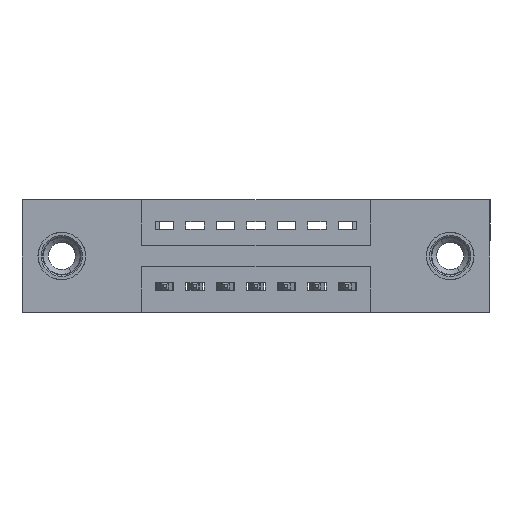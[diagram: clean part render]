
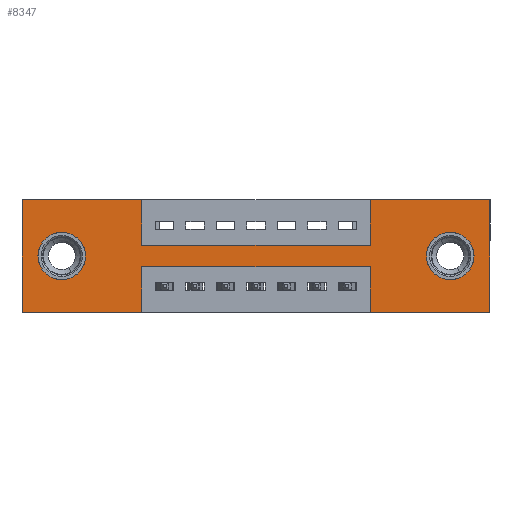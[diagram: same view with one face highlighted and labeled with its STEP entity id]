
A CAD part, front view. The second image highlights one B-rep face of the part: STEP entity #8347.
In plain terms, the highlighted planar face has unit normal (0, -1, 0).
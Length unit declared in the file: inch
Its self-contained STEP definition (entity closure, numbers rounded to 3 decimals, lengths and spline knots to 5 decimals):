
#15 = CARTESIAN_POINT ( 'NONE',  ( 1.405, 0., -0.263 ) ) ;
#103 = CARTESIAN_POINT ( 'NONE',  ( 1.1425, 0., -0.37 ) ) ;
#186 = DIRECTION ( 'NONE',  ( 0., 0., 1. ) ) ;
#274 = CARTESIAN_POINT ( 'NONE',  ( 1.1425, 0., -0.22 ) ) ;
#334 = DIRECTION ( 'NONE',  ( 0., 1., 0. ) ) ;
#341 = DIRECTION ( 'NONE',  ( 0., 1., 0. ) ) ;
#422 = CARTESIAN_POINT ( 'NONE',  ( 1.405, 0., -0.185 ) ) ;
#465 = DIRECTION ( 'NONE',  ( 0., 1., 0. ) ) ;
#527 = ORIENTED_EDGE ( 'NONE', *, *, #3583, .F. ) ;
#692 = VERTEX_POINT ( 'NONE', #10592 ) ;
#693 = ORIENTED_EDGE ( 'NONE', *, *, #2341, .F. ) ;
#712 = ORIENTED_EDGE ( 'NONE', *, *, #7673, .F. ) ;
#758 = DIRECTION ( 'NONE',  ( -1., 0., 0. ) ) ;
#780 = ORIENTED_EDGE ( 'NONE', *, *, #11427, .F. ) ;
#804 = ORIENTED_EDGE ( 'NONE', *, *, #12140, .F. ) ;
#953 = VECTOR ( 'NONE', #7619, 39.37008 ) ;
#972 = CARTESIAN_POINT ( 'NONE',  ( 0., 0., 0. ) ) ;
#1027 = DIRECTION ( 'NONE',  ( 0., 0., -1. ) ) ;
#1092 = ORIENTED_EDGE ( 'NONE', *, *, #7418, .T. ) ;
#1147 = VERTEX_POINT ( 'NONE', #6184 ) ;
#1318 = VERTEX_POINT ( 'NONE', #2509 ) ;
#1420 = ORIENTED_EDGE ( 'NONE', *, *, #5112, .F. ) ;
#1443 = CARTESIAN_POINT ( 'NONE',  ( 0.13, 0., -0.185 ) ) ;
#1456 = AXIS2_PLACEMENT_3D ( 'NONE', #2795, #9388, #11253 ) ;
#1524 = LINE ( 'NONE', #972, #10943 ) ;
#1564 = DIRECTION ( 'NONE',  ( -1., 0., 0. ) ) ;
#1749 = EDGE_CURVE ( 'NONE', #9390, #4293, #10101, .T. ) ;
#1927 = DIRECTION ( 'NONE',  ( 1., 0., 0. ) ) ;
#1957 = CARTESIAN_POINT ( 'NONE',  ( 0., 0., 0. ) ) ;
#1993 = LINE ( 'NONE', #1957, #953 ) ;
#2012 = LINE ( 'NONE', #10141, #4493 ) ;
#2042 = CARTESIAN_POINT ( 'NONE',  ( 0.3925, 0., -0.37 ) ) ;
#2138 = CARTESIAN_POINT ( 'NONE',  ( 1.1425, 0., -0.37 ) ) ;
#2214 = LINE ( 'NONE', #8931, #7953 ) ;
#2218 = ORIENTED_EDGE ( 'NONE', *, *, #7814, .T. ) ;
#2341 = EDGE_CURVE ( 'NONE', #6186, #4731, #8759, .T. ) ;
#2509 = CARTESIAN_POINT ( 'NONE',  ( 0.3925, 0., -0.15 ) ) ;
#2535 = CARTESIAN_POINT ( 'NONE',  ( 0., 0., -0.37 ) ) ;
#2539 = CARTESIAN_POINT ( 'NONE',  ( 1.1425, 0., 0. ) ) ;
#2795 = CARTESIAN_POINT ( 'NONE',  ( 0., 0., -0.37 ) ) ;
#2875 = VECTOR ( 'NONE', #8533, 39.37008 ) ;
#2930 = EDGE_LOOP ( 'NONE', ( #6854, #8489, #693, #527, #804, #712, #3038, #780, #1420, #8647, #11917, #7515 ) ) ;
#3038 = ORIENTED_EDGE ( 'NONE', *, *, #9083, .F. ) ;
#3223 = CARTESIAN_POINT ( 'NONE',  ( 0.13, 0., -0.185 ) ) ;
#3583 = EDGE_CURVE ( 'NONE', #1147, #6186, #9122, .T. ) ;
#3720 = CARTESIAN_POINT ( 'NONE',  ( 0., 0., -0.37 ) ) ;
#3762 = CARTESIAN_POINT ( 'NONE',  ( 1.535, 0., 0. ) ) ;
#4062 = LINE ( 'NONE', #7671, #9357 ) ;
#4078 = DIRECTION ( 'NONE',  ( 0., 0., 1. ) ) ;
#4095 = EDGE_CURVE ( 'NONE', #9606, #11121, #4566, .T. ) ;
#4162 = CIRCLE ( 'NONE', #8846, 0.078 ) ;
#4177 = CIRCLE ( 'NONE', #8293, 0.078 ) ;
#4293 = VERTEX_POINT ( 'NONE', #7997 ) ;
#4306 = DIRECTION ( 'NONE',  ( 0., 0., -1. ) ) ;
#4493 = VECTOR ( 'NONE', #758, 39.37008 ) ;
#4566 = CIRCLE ( 'NONE', #11667, 0.078 ) ;
#4603 = LINE ( 'NONE', #12172, #8989 ) ;
#4631 = DIRECTION ( 'NONE',  ( 0., 0., 1. ) ) ;
#4708 = VERTEX_POINT ( 'NONE', #15 ) ;
#4731 = VERTEX_POINT ( 'NONE', #274 ) ;
#4895 = CARTESIAN_POINT ( 'NONE',  ( 0.3925, 0., -0.22 ) ) ;
#5112 = EDGE_CURVE ( 'NONE', #5914, #1318, #6029, .T. ) ;
#5321 = CARTESIAN_POINT ( 'NONE',  ( 0., 0., 0. ) ) ;
#5438 = CARTESIAN_POINT ( 'NONE',  ( 0., 0., 0. ) ) ;
#5441 = VECTOR ( 'NONE', #1564, 39.37008 ) ;
#5484 = CARTESIAN_POINT ( 'NONE',  ( 1.1425, 0., -0.15 ) ) ;
#5727 = VECTOR ( 'NONE', #1027, 39.37008 ) ;
#5738 = LINE ( 'NONE', #3762, #8076 ) ;
#5914 = VERTEX_POINT ( 'NONE', #10557 ) ;
#5963 = VECTOR ( 'NONE', #186, 39.37008 ) ;
#5968 = CARTESIAN_POINT ( 'NONE',  ( 1.405, 0., -0.185 ) ) ;
#6029 = LINE ( 'NONE', #8507, #5727 ) ;
#6184 = CARTESIAN_POINT ( 'NONE',  ( 1.535, 0., -0.37 ) ) ;
#6186 = VERTEX_POINT ( 'NONE', #2138 ) ;
#6219 = CARTESIAN_POINT ( 'NONE',  ( 0.13, 0., -0.107 ) ) ;
#6510 = EDGE_CURVE ( 'NONE', #4731, #9714, #2012, .T. ) ;
#6512 = FACE_OUTER_BOUND ( 'NONE', #2930, .T. ) ;
#6676 = EDGE_CURVE ( 'NONE', #9714, #9390, #4062, .T. ) ;
#6747 = EDGE_LOOP ( 'NONE', ( #1092, #8422 ) ) ;
#6854 = ORIENTED_EDGE ( 'NONE', *, *, #6676, .F. ) ;
#7052 = VERTEX_POINT ( 'NONE', #5321 ) ;
#7059 = EDGE_CURVE ( 'NONE', #4293, #7052, #7744, .T. ) ;
#7104 = FACE_BOUND ( 'NONE', #11002, .T. ) ;
#7418 = EDGE_CURVE ( 'NONE', #11121, #9606, #4177, .T. ) ;
#7469 = PLANE ( 'NONE',  #1456 ) ;
#7515 = ORIENTED_EDGE ( 'NONE', *, *, #1749, .F. ) ;
#7619 = DIRECTION ( 'NONE',  ( 1., 0., 0. ) ) ;
#7671 = CARTESIAN_POINT ( 'NONE',  ( 0.3925, 0., -0.37 ) ) ;
#7673 = EDGE_CURVE ( 'NONE', #11431, #11813, #1993, .T. ) ;
#7744 = LINE ( 'NONE', #5438, #9032 ) ;
#7814 = EDGE_CURVE ( 'NONE', #692, #4708, #4162, .T. ) ;
#7857 = DIRECTION ( 'NONE',  ( 0., 0., -1. ) ) ;
#7920 = EDGE_CURVE ( 'NONE', #7052, #5914, #1524, .T. ) ;
#7953 = VECTOR ( 'NONE', #10803, 39.37008 ) ;
#7983 = CARTESIAN_POINT ( 'NONE',  ( 0.13, 0., -0.263 ) ) ;
#7997 = CARTESIAN_POINT ( 'NONE',  ( 0., 0., -0.37 ) ) ;
#8076 = VECTOR ( 'NONE', #9401, 39.37008 ) ;
#8293 = AXIS2_PLACEMENT_3D ( 'NONE', #1443, #341, #4078 ) ;
#8347 = ADVANCED_FACE ( 'NONE', ( #7104, #10488, #6512 ), #7469, .T. ) ;
#8422 = ORIENTED_EDGE ( 'NONE', *, *, #4095, .T. ) ;
#8489 = ORIENTED_EDGE ( 'NONE', *, *, #6510, .F. ) ;
#8507 = CARTESIAN_POINT ( 'NONE',  ( 0.3925, 0., 0. ) ) ;
#8533 = DIRECTION ( 'NONE',  ( -1., 0., 0. ) ) ;
#8647 = ORIENTED_EDGE ( 'NONE', *, *, #7920, .F. ) ;
#8759 = LINE ( 'NONE', #103, #5963 ) ;
#8846 = AXIS2_PLACEMENT_3D ( 'NONE', #422, #465, #4306 ) ;
#8931 = CARTESIAN_POINT ( 'NONE',  ( 0.3925, 0., -0.15 ) ) ;
#8989 = VECTOR ( 'NONE', #4631, 39.37008 ) ;
#9032 = VECTOR ( 'NONE', #12021, 39.37008 ) ;
#9083 = EDGE_CURVE ( 'NONE', #12078, #11431, #4603, .T. ) ;
#9122 = LINE ( 'NONE', #2535, #5441 ) ;
#9310 = CIRCLE ( 'NONE', #11406, 0.078 ) ;
#9357 = VECTOR ( 'NONE', #11537, 39.37008 ) ;
#9388 = DIRECTION ( 'NONE',  ( 0., -1., 0. ) ) ;
#9390 = VERTEX_POINT ( 'NONE', #2042 ) ;
#9401 = DIRECTION ( 'NONE',  ( 0., 0., -1. ) ) ;
#9606 = VERTEX_POINT ( 'NONE', #7983 ) ;
#9714 = VERTEX_POINT ( 'NONE', #4895 ) ;
#9829 = DIRECTION ( 'NONE',  ( 0., 0., 1. ) ) ;
#9949 = DIRECTION ( 'NONE',  ( 0., 1., 0. ) ) ;
#10101 = LINE ( 'NONE', #3720, #2875 ) ;
#10141 = CARTESIAN_POINT ( 'NONE',  ( 0.3925, 0., -0.22 ) ) ;
#10439 = EDGE_CURVE ( 'NONE', #4708, #692, #9310, .T. ) ;
#10488 = FACE_BOUND ( 'NONE', #6747, .T. ) ;
#10557 = CARTESIAN_POINT ( 'NONE',  ( 0.3925, 0., 0. ) ) ;
#10592 = CARTESIAN_POINT ( 'NONE',  ( 1.405, 0., -0.107 ) ) ;
#10690 = CARTESIAN_POINT ( 'NONE',  ( 1.535, 0., 0. ) ) ;
#10803 = DIRECTION ( 'NONE',  ( 1., 0., 0. ) ) ;
#10943 = VECTOR ( 'NONE', #1927, 39.37008 ) ;
#11002 = EDGE_LOOP ( 'NONE', ( #2218, #11160 ) ) ;
#11121 = VERTEX_POINT ( 'NONE', #6219 ) ;
#11160 = ORIENTED_EDGE ( 'NONE', *, *, #10439, .T. ) ;
#11253 = DIRECTION ( 'NONE',  ( 0., 0., -1. ) ) ;
#11406 = AXIS2_PLACEMENT_3D ( 'NONE', #5968, #334, #7857 ) ;
#11427 = EDGE_CURVE ( 'NONE', #1318, #12078, #2214, .T. ) ;
#11431 = VERTEX_POINT ( 'NONE', #2539 ) ;
#11537 = DIRECTION ( 'NONE',  ( 0., 0., -1. ) ) ;
#11667 = AXIS2_PLACEMENT_3D ( 'NONE', #3223, #9949, #9829 ) ;
#11813 = VERTEX_POINT ( 'NONE', #10690 ) ;
#11917 = ORIENTED_EDGE ( 'NONE', *, *, #7059, .F. ) ;
#12021 = DIRECTION ( 'NONE',  ( 0., 0., 1. ) ) ;
#12078 = VERTEX_POINT ( 'NONE', #5484 ) ;
#12140 = EDGE_CURVE ( 'NONE', #11813, #1147, #5738, .T. ) ;
#12172 = CARTESIAN_POINT ( 'NONE',  ( 1.1425, 0., 0. ) ) ;
